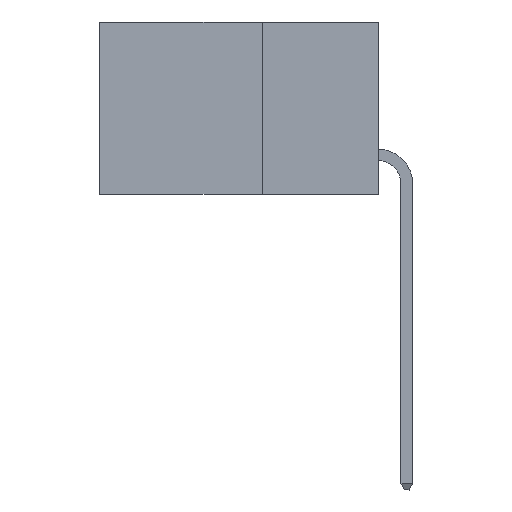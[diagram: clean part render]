
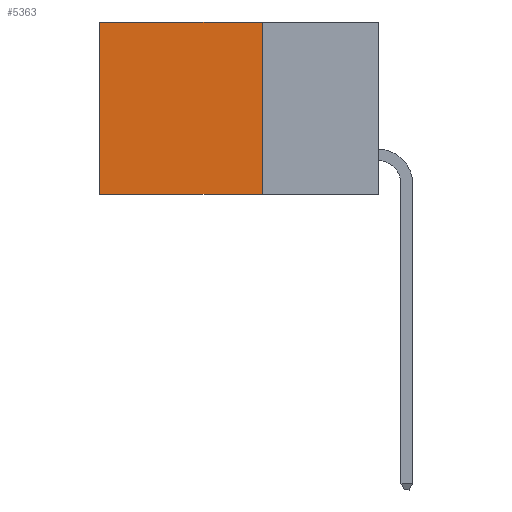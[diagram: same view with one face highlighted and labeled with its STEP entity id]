
A CAD part, left-side view. The second image highlights one B-rep face of the part: STEP entity #5363.
In plain terms, the highlighted planar face has unit normal (-1, 0, 0).
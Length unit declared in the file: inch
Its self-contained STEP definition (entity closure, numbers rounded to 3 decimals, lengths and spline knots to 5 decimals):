
#99 = DIRECTION ( 'NONE',  ( 0., 1., 0. ) ) ;
#853 = VECTOR ( 'NONE', #6342, 39.37008 ) ;
#1045 = ORIENTED_EDGE ( 'NONE', *, *, #5316, .F. ) ;
#1776 = VECTOR ( 'NONE', #99, 39.37008 ) ;
#1962 = CARTESIAN_POINT ( 'NONE',  ( 0.2615, 0.6, -0.37 ) ) ;
#2475 = CARTESIAN_POINT ( 'NONE',  ( 0.2615, 0.25, -0.37 ) ) ;
#2693 = VERTEX_POINT ( 'NONE', #1962 ) ;
#2790 = VERTEX_POINT ( 'NONE', #6703 ) ;
#3922 = EDGE_CURVE ( 'NONE', #12255, #2693, #10727, .T. ) ;
#5105 = CARTESIAN_POINT ( 'NONE',  ( 0.2615, 0.6, -0.37 ) ) ;
#5316 = EDGE_CURVE ( 'NONE', #2790, #9819, #8772, .T. ) ;
#5363 = ADVANCED_FACE ( 'NONE', ( #8224 ), #5973, .F. ) ;
#5396 = AXIS2_PLACEMENT_3D ( 'NONE', #2475, #10495, #7946 ) ;
#5633 = VECTOR ( 'NONE', #13233, 39.37008 ) ;
#5777 = DIRECTION ( 'NONE',  ( 0., 1., 0. ) ) ;
#5787 = EDGE_LOOP ( 'NONE', ( #14084, #7287, #1045, #6948 ) ) ;
#5973 = PLANE ( 'NONE',  #5396 ) ;
#6217 = CARTESIAN_POINT ( 'NONE',  ( 0.2615, 0.6, 0. ) ) ;
#6342 = DIRECTION ( 'NONE',  ( 0., 0., -1. ) ) ;
#6586 = CARTESIAN_POINT ( 'NONE',  ( 0.2615, 0.25, -0.37 ) ) ;
#6703 = CARTESIAN_POINT ( 'NONE',  ( 0.2615, 0.25, 0. ) ) ;
#6948 = ORIENTED_EDGE ( 'NONE', *, *, #11886, .T. ) ;
#7287 = ORIENTED_EDGE ( 'NONE', *, *, #13788, .F. ) ;
#7946 = DIRECTION ( 'NONE',  ( 0., 0., -1. ) ) ;
#8224 = FACE_OUTER_BOUND ( 'NONE', #5787, .T. ) ;
#8772 = LINE ( 'NONE', #8991, #5633 ) ;
#8991 = CARTESIAN_POINT ( 'NONE',  ( 0.2615, 0.25, -0.37 ) ) ;
#9222 = LINE ( 'NONE', #13667, #11128 ) ;
#9819 = VERTEX_POINT ( 'NONE', #6586 ) ;
#10495 = DIRECTION ( 'NONE',  ( 1., 0., 0. ) ) ;
#10727 = LINE ( 'NONE', #5105, #853 ) ;
#11055 = CARTESIAN_POINT ( 'NONE',  ( 0.2615, 0.25, 0. ) ) ;
#11128 = VECTOR ( 'NONE', #5777, 39.37008 ) ;
#11886 = EDGE_CURVE ( 'NONE', #2790, #12255, #13544, .T. ) ;
#12255 = VERTEX_POINT ( 'NONE', #6217 ) ;
#13233 = DIRECTION ( 'NONE',  ( 0., 0., -1. ) ) ;
#13544 = LINE ( 'NONE', #11055, #1776 ) ;
#13667 = CARTESIAN_POINT ( 'NONE',  ( 0.2615, 0.25, -0.37 ) ) ;
#13788 = EDGE_CURVE ( 'NONE', #9819, #2693, #9222, .T. ) ;
#14084 = ORIENTED_EDGE ( 'NONE', *, *, #3922, .T. ) ;
